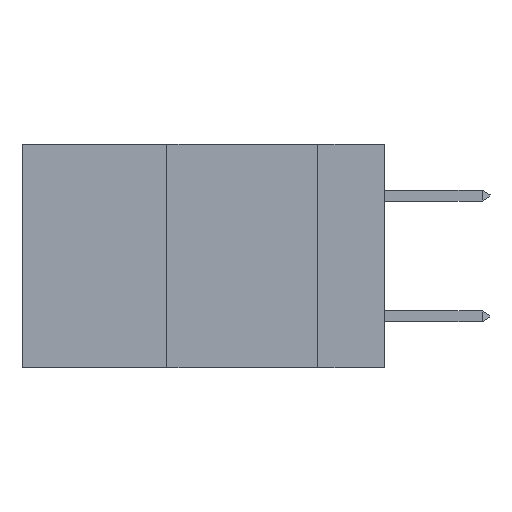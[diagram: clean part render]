
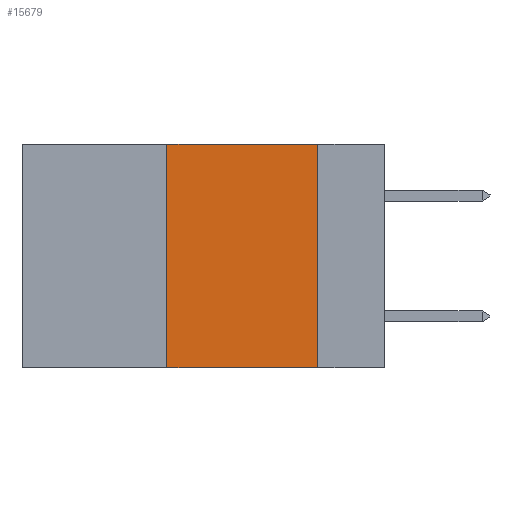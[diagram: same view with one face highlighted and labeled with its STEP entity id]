
A CAD part, left-side view. The second image highlights one B-rep face of the part: STEP entity #15679.
In plain terms, the highlighted planar face has unit normal (-1, 0, 0).
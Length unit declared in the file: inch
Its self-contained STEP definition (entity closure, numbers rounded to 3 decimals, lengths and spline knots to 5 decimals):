
#542 = CARTESIAN_POINT ( 'NONE',  ( 0., 0.36, 0. ) ) ;
#814 = VECTOR ( 'NONE', #21250, 39.37008 ) ;
#927 = ORIENTED_EDGE ( 'NONE', *, *, #38491, .F. ) ;
#3169 = EDGE_CURVE ( 'NONE', #36343, #29320, #19176, .T. ) ;
#5494 = CARTESIAN_POINT ( 'NONE',  ( 0., 0.36, 0. ) ) ;
#7402 = ORIENTED_EDGE ( 'NONE', *, *, #18266, .F. ) ;
#8941 = DIRECTION ( 'NONE',  ( 0., -1., 0. ) ) ;
#9121 = CARTESIAN_POINT ( 'NONE',  ( 0., 0.11, 0. ) ) ;
#9924 = CARTESIAN_POINT ( 'NONE',  ( 0., 0.6, -0.37 ) ) ;
#11131 = DIRECTION ( 'NONE',  ( 0., 0., -1. ) ) ;
#11765 = CARTESIAN_POINT ( 'NONE',  ( 0., 0.6, 0. ) ) ;
#13072 = DIRECTION ( 'NONE',  ( 0., -1., 0. ) ) ;
#14503 = PLANE ( 'NONE',  #36204 ) ;
#15679 = ADVANCED_FACE ( 'NONE', ( #40499 ), #14503, .F. ) ;
#18266 = EDGE_CURVE ( 'NONE', #36343, #28945, #21465, .T. ) ;
#18416 = VECTOR ( 'NONE', #29926, 39.37008 ) ;
#19176 = LINE ( 'NONE', #9924, #32106 ) ;
#19240 = EDGE_LOOP ( 'NONE', ( #927, #32846, #7402, #22360 ) ) ;
#19657 = VERTEX_POINT ( 'NONE', #9121 ) ;
#20156 = CARTESIAN_POINT ( 'NONE',  ( 0., 0.36, -0.37 ) ) ;
#20398 = DIRECTION ( 'NONE',  ( 1., 0., 0. ) ) ;
#20476 = CARTESIAN_POINT ( 'NONE',  ( 0., 0.11, 0. ) ) ;
#21250 = DIRECTION ( 'NONE',  ( 0., 0., 1. ) ) ;
#21465 = LINE ( 'NONE', #5494, #814 ) ;
#21773 = CARTESIAN_POINT ( 'NONE',  ( 0., 0.6, 0. ) ) ;
#21782 = VECTOR ( 'NONE', #8941, 39.37008 ) ;
#22360 = ORIENTED_EDGE ( 'NONE', *, *, #3169, .T. ) ;
#25112 = LINE ( 'NONE', #21773, #21782 ) ;
#28945 = VERTEX_POINT ( 'NONE', #542 ) ;
#29320 = VERTEX_POINT ( 'NONE', #32425 ) ;
#29926 = DIRECTION ( 'NONE',  ( 0., 0., -1. ) ) ;
#32106 = VECTOR ( 'NONE', #13072, 39.37008 ) ;
#32425 = CARTESIAN_POINT ( 'NONE',  ( 0., 0.11, -0.37 ) ) ;
#32846 = ORIENTED_EDGE ( 'NONE', *, *, #38213, .F. ) ;
#36204 = AXIS2_PLACEMENT_3D ( 'NONE', #11765, #20398, #11131 ) ;
#36343 = VERTEX_POINT ( 'NONE', #20156 ) ;
#36610 = LINE ( 'NONE', #20476, #18416 ) ;
#38213 = EDGE_CURVE ( 'NONE', #28945, #19657, #25112, .T. ) ;
#38491 = EDGE_CURVE ( 'NONE', #19657, #29320, #36610, .T. ) ;
#40499 = FACE_OUTER_BOUND ( 'NONE', #19240, .T. ) ;
